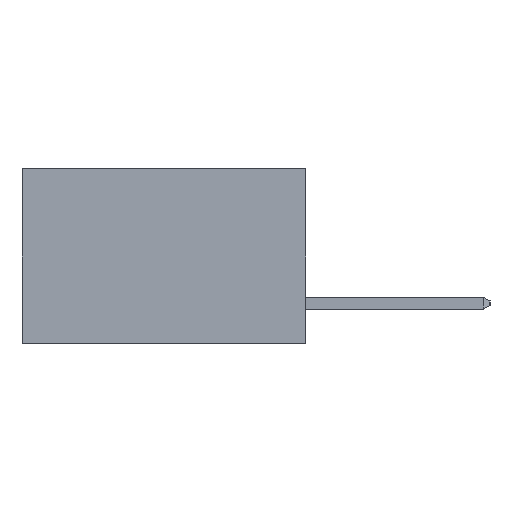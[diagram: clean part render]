
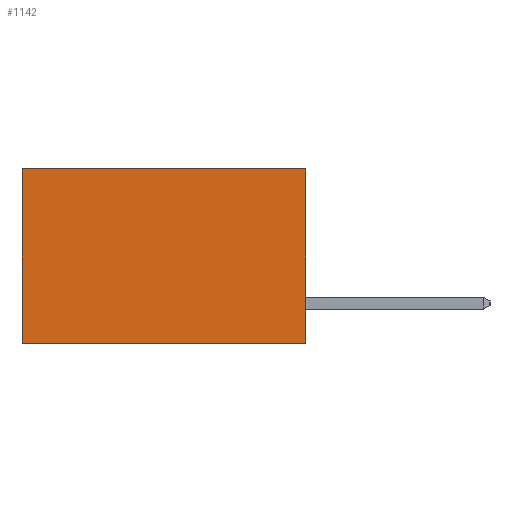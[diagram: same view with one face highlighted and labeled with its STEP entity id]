
A CAD part, left-side view. The second image highlights one B-rep face of the part: STEP entity #1142.
In plain terms, the highlighted planar face has unit normal (-1, 0, 0).
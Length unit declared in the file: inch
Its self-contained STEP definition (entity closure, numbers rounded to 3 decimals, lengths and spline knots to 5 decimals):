
#344 = DIRECTION ( 'NONE',  ( 0., 1., 0. ) ) ;
#871 = EDGE_CURVE ( 'NONE', #12426, #21276, #3186, .T. ) ;
#1075 = LINE ( 'NONE', #5730, #19274 ) ;
#1142 = ADVANCED_FACE ( 'NONE', ( #9008 ), #13356, .F. ) ;
#3186 = LINE ( 'NONE', #15988, #20674 ) ;
#4676 = VERTEX_POINT ( 'NONE', #19196 ) ;
#4694 = VECTOR ( 'NONE', #19163, 39.37008 ) ;
#5588 = VECTOR ( 'NONE', #13046, 39.37008 ) ;
#5730 = CARTESIAN_POINT ( 'NONE',  ( 0.2615, 0.6, -0.37 ) ) ;
#5841 = CARTESIAN_POINT ( 'NONE',  ( 0.2615, 0., -0.37 ) ) ;
#8787 = ORIENTED_EDGE ( 'NONE', *, *, #17431, .F. ) ;
#9008 = FACE_OUTER_BOUND ( 'NONE', #21803, .T. ) ;
#9110 = DIRECTION ( 'NONE',  ( 0., 0., -1. ) ) ;
#10155 = LINE ( 'NONE', #18182, #5588 ) ;
#11085 = AXIS2_PLACEMENT_3D ( 'NONE', #13314, #13281, #13265 ) ;
#12426 = VERTEX_POINT ( 'NONE', #5841 ) ;
#12691 = ORIENTED_EDGE ( 'NONE', *, *, #19754, .T. ) ;
#12984 = ORIENTED_EDGE ( 'NONE', *, *, #871, .F. ) ;
#13046 = DIRECTION ( 'NONE',  ( 0., 1., 0. ) ) ;
#13265 = DIRECTION ( 'NONE',  ( 0., 0., -1. ) ) ;
#13281 = DIRECTION ( 'NONE',  ( 1., 0., 0. ) ) ;
#13314 = CARTESIAN_POINT ( 'NONE',  ( 0.2615, 0., -0.37 ) ) ;
#13356 = PLANE ( 'NONE',  #11085 ) ;
#15006 = EDGE_CURVE ( 'NONE', #4676, #16566, #10155, .T. ) ;
#15988 = CARTESIAN_POINT ( 'NONE',  ( 0.2615, 0., -0.37 ) ) ;
#16566 = VERTEX_POINT ( 'NONE', #18767 ) ;
#17431 = EDGE_CURVE ( 'NONE', #4676, #12426, #18334, .T. ) ;
#17508 = CARTESIAN_POINT ( 'NONE',  ( 0.2615, 0., -0.37 ) ) ;
#18182 = CARTESIAN_POINT ( 'NONE',  ( 0.2615, 0., 0. ) ) ;
#18334 = LINE ( 'NONE', #17508, #4694 ) ;
#18767 = CARTESIAN_POINT ( 'NONE',  ( 0.2615, 0.6, 0. ) ) ;
#19163 = DIRECTION ( 'NONE',  ( 0., 0., -1. ) ) ;
#19196 = CARTESIAN_POINT ( 'NONE',  ( 0.2615, 0., 0. ) ) ;
#19274 = VECTOR ( 'NONE', #9110, 39.37008 ) ;
#19588 = CARTESIAN_POINT ( 'NONE',  ( 0.2615, 0.6, -0.37 ) ) ;
#19754 = EDGE_CURVE ( 'NONE', #16566, #21276, #1075, .T. ) ;
#20674 = VECTOR ( 'NONE', #344, 39.37008 ) ;
#21276 = VERTEX_POINT ( 'NONE', #19588 ) ;
#21803 = EDGE_LOOP ( 'NONE', ( #12691, #12984, #8787, #21991 ) ) ;
#21991 = ORIENTED_EDGE ( 'NONE', *, *, #15006, .T. ) ;
